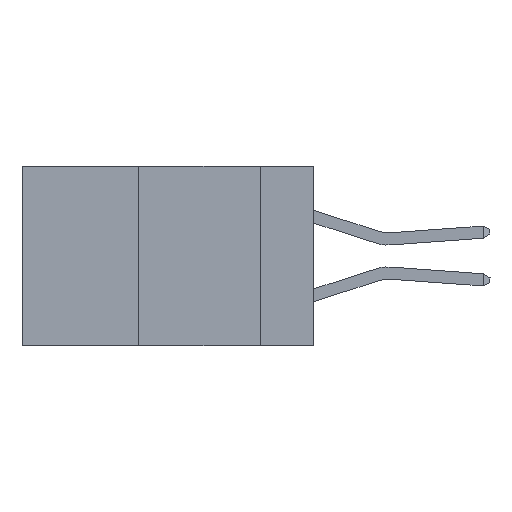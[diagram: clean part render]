
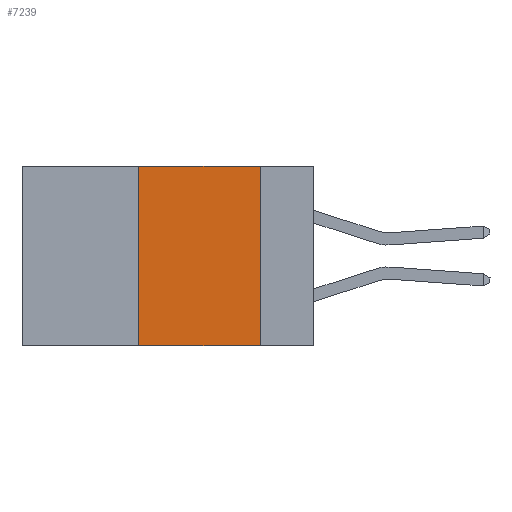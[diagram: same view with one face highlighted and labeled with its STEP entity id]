
A CAD part, left-side view. The second image highlights one B-rep face of the part: STEP entity #7239.
In plain terms, the highlighted planar face has unit normal (-1, 0, 0).
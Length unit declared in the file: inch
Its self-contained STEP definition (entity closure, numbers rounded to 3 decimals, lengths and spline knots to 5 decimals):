
#717 = FACE_OUTER_BOUND ( 'NONE', #9328, .T. ) ;
#1005 = ORIENTED_EDGE ( 'NONE', *, *, #5696, .T. ) ;
#1088 = ORIENTED_EDGE ( 'NONE', *, *, #10741, .F. ) ;
#2277 = CARTESIAN_POINT ( 'NONE',  ( 0., 0.11, 0. ) ) ;
#2302 = ORIENTED_EDGE ( 'NONE', *, *, #14799, .F. ) ;
#2583 = VERTEX_POINT ( 'NONE', #3182 ) ;
#2768 = VERTEX_POINT ( 'NONE', #2277 ) ;
#3182 = CARTESIAN_POINT ( 'NONE',  ( 0., 0.36, 0. ) ) ;
#3422 = ORIENTED_EDGE ( 'NONE', *, *, #5839, .F. ) ;
#4195 = AXIS2_PLACEMENT_3D ( 'NONE', #5259, #15125, #7793 ) ;
#4382 = CARTESIAN_POINT ( 'NONE',  ( 0., 0.11, 0. ) ) ;
#5259 = CARTESIAN_POINT ( 'NONE',  ( 0., 0.6, 0. ) ) ;
#5696 = EDGE_CURVE ( 'NONE', #7183, #8913, #6831, .T. ) ;
#5839 = EDGE_CURVE ( 'NONE', #2583, #2768, #14356, .T. ) ;
#6428 = VECTOR ( 'NONE', #14716, 39.37008 ) ;
#6431 = CARTESIAN_POINT ( 'NONE',  ( 0., 0.36, -0.37 ) ) ;
#6524 = VECTOR ( 'NONE', #10785, 39.37008 ) ;
#6831 = LINE ( 'NONE', #12242, #6428 ) ;
#7183 = VERTEX_POINT ( 'NONE', #6431 ) ;
#7239 = ADVANCED_FACE ( 'NONE', ( #717 ), #13944, .F. ) ;
#7408 = VECTOR ( 'NONE', #12604, 39.37008 ) ;
#7793 = DIRECTION ( 'NONE',  ( 0., 0., -1. ) ) ;
#8686 = CARTESIAN_POINT ( 'NONE',  ( 0., 0.36, 0. ) ) ;
#8800 = CARTESIAN_POINT ( 'NONE',  ( 0., 0.11, -0.37 ) ) ;
#8913 = VERTEX_POINT ( 'NONE', #8800 ) ;
#9328 = EDGE_LOOP ( 'NONE', ( #2302, #3422, #1088, #1005 ) ) ;
#9853 = LINE ( 'NONE', #4382, #6524 ) ;
#9945 = DIRECTION ( 'NONE',  ( 0., 0., 1. ) ) ;
#10141 = CARTESIAN_POINT ( 'NONE',  ( 0., 0.6, 0. ) ) ;
#10741 = EDGE_CURVE ( 'NONE', #7183, #2583, #14771, .T. ) ;
#10785 = DIRECTION ( 'NONE',  ( 0., 0., -1. ) ) ;
#12242 = CARTESIAN_POINT ( 'NONE',  ( 0., 0.6, -0.37 ) ) ;
#12604 = DIRECTION ( 'NONE',  ( 0., -1., 0. ) ) ;
#13944 = PLANE ( 'NONE',  #4195 ) ;
#14356 = LINE ( 'NONE', #10141, #7408 ) ;
#14716 = DIRECTION ( 'NONE',  ( 0., -1., 0. ) ) ;
#14771 = LINE ( 'NONE', #8686, #15121 ) ;
#14799 = EDGE_CURVE ( 'NONE', #2768, #8913, #9853, .T. ) ;
#15121 = VECTOR ( 'NONE', #9945, 39.37008 ) ;
#15125 = DIRECTION ( 'NONE',  ( 1., 0., 0. ) ) ;
